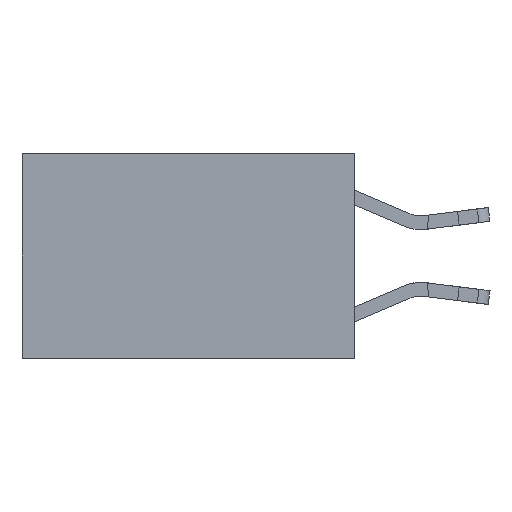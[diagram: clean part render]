
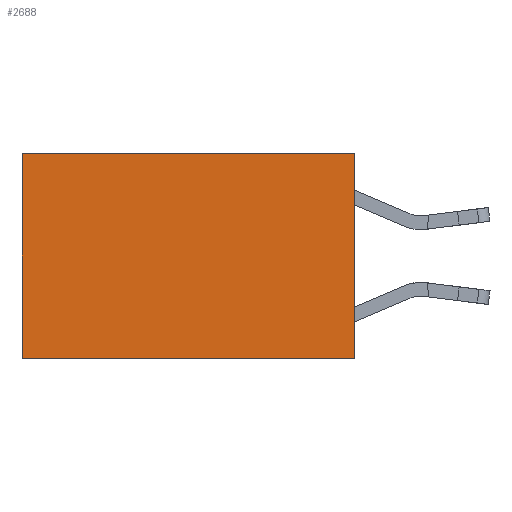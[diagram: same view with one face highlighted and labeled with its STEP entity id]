
A CAD part, left-side view. The second image highlights one B-rep face of the part: STEP entity #2688.
In plain terms, the highlighted planar face has unit normal (-1, 0, 0).
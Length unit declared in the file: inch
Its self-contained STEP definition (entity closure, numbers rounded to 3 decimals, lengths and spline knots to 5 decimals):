
#1319 = DIRECTION ( 'NONE',  ( 0., 0., -1. ) ) ;
#1782 = VECTOR ( 'NONE', #10608, 39.37008 ) ;
#2366 = DIRECTION ( 'NONE',  ( 0., 1., 0. ) ) ;
#2688 = ADVANCED_FACE ( 'NONE', ( #12695 ), #5232, .F. ) ;
#2831 = LINE ( 'NONE', #19249, #8030 ) ;
#3450 = CARTESIAN_POINT ( 'NONE',  ( 0.2625, 0., -0.37 ) ) ;
#3740 = VERTEX_POINT ( 'NONE', #7739 ) ;
#4049 = VERTEX_POINT ( 'NONE', #17267 ) ;
#4391 = VECTOR ( 'NONE', #2366, 39.37008 ) ;
#5133 = DIRECTION ( 'NONE',  ( 1., 0., 0. ) ) ;
#5232 = PLANE ( 'NONE',  #13940 ) ;
#6291 = EDGE_CURVE ( 'NONE', #12963, #4049, #16986, .T. ) ;
#6523 = LINE ( 'NONE', #12600, #1782 ) ;
#7739 = CARTESIAN_POINT ( 'NONE',  ( 0.2625, 0., 0. ) ) ;
#7743 = ORIENTED_EDGE ( 'NONE', *, *, #11057, .T. ) ;
#8030 = VECTOR ( 'NONE', #1319, 39.37008 ) ;
#8533 = CARTESIAN_POINT ( 'NONE',  ( 0.2625, 0., 0. ) ) ;
#9590 = ORIENTED_EDGE ( 'NONE', *, *, #10005, .F. ) ;
#10005 = EDGE_CURVE ( 'NONE', #3740, #12963, #6523, .T. ) ;
#10608 = DIRECTION ( 'NONE',  ( 0., 0., -1. ) ) ;
#11057 = EDGE_CURVE ( 'NONE', #3740, #14471, #16082, .T. ) ;
#11200 = DIRECTION ( 'NONE',  ( 0., 0., -1. ) ) ;
#11539 = ORIENTED_EDGE ( 'NONE', *, *, #14120, .T. ) ;
#11873 = CARTESIAN_POINT ( 'NONE',  ( 0.2625, 0.6, 0. ) ) ;
#12600 = CARTESIAN_POINT ( 'NONE',  ( 0.2625, 0., 0. ) ) ;
#12695 = FACE_OUTER_BOUND ( 'NONE', #16601, .T. ) ;
#12963 = VERTEX_POINT ( 'NONE', #3450 ) ;
#13940 = AXIS2_PLACEMENT_3D ( 'NONE', #18763, #5133, #11200 ) ;
#14120 = EDGE_CURVE ( 'NONE', #14471, #4049, #2831, .T. ) ;
#14471 = VERTEX_POINT ( 'NONE', #11873 ) ;
#15170 = DIRECTION ( 'NONE',  ( 0., 1., 0. ) ) ;
#15394 = ORIENTED_EDGE ( 'NONE', *, *, #6291, .F. ) ;
#16082 = LINE ( 'NONE', #8533, #4391 ) ;
#16601 = EDGE_LOOP ( 'NONE', ( #11539, #15394, #9590, #7743 ) ) ;
#16871 = VECTOR ( 'NONE', #15170, 39.37008 ) ;
#16986 = LINE ( 'NONE', #18574, #16871 ) ;
#17267 = CARTESIAN_POINT ( 'NONE',  ( 0.2625, 0.6, -0.37 ) ) ;
#18574 = CARTESIAN_POINT ( 'NONE',  ( 0.2625, 0., -0.37 ) ) ;
#18763 = CARTESIAN_POINT ( 'NONE',  ( 0.2625, 0., 0. ) ) ;
#19249 = CARTESIAN_POINT ( 'NONE',  ( 0.2625, 0.6, 0. ) ) ;
